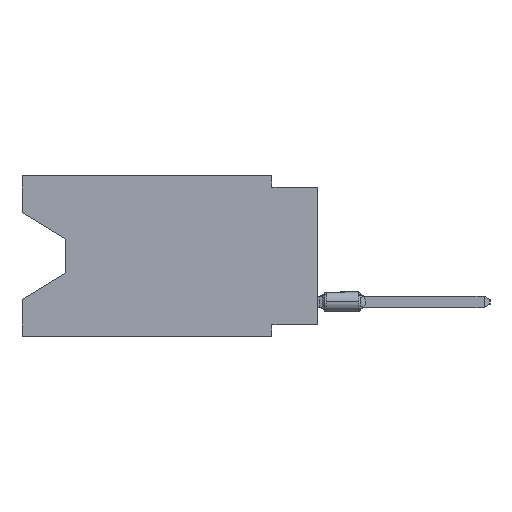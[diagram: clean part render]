
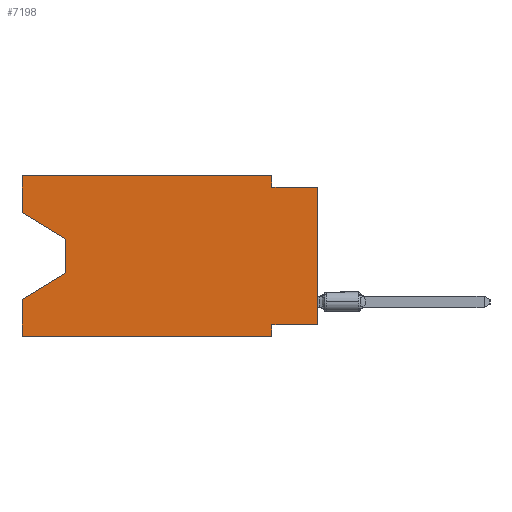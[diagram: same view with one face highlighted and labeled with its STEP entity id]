
A CAD part, left-side view. The second image highlights one B-rep face of the part: STEP entity #7198.
In plain terms, the highlighted planar face has unit normal (-1, 0, 0).
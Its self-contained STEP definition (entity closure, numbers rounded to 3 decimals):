
#345 = EDGE_LOOP ( 'NONE', ( #53610, #30509, #51926, #1708, #21597, #31156, #34441, #54796, #28527, #40102, #48692, #1842 ) ) ;
#1117 = EDGE_CURVE ( 'NONE', #38565, #13329, #57791, .T. ) ;
#1708 = ORIENTED_EDGE ( 'NONE', *, *, #26189, .F. ) ;
#1778 = CARTESIAN_POINT ( 'NONE',  ( 0., 16.383, -2.038 ) ) ;
#1842 = ORIENTED_EDGE ( 'NONE', *, *, #42715, .F. ) ;
#1951 = VECTOR ( 'NONE', #3642, 1000. ) ;
#2028 = VERTEX_POINT ( 'NONE', #43649 ) ;
#2333 = AXIS2_PLACEMENT_3D ( 'NONE', #37307, #8423, #46614 ) ;
#3642 = DIRECTION ( 'NONE',  ( 0., 0., 1. ) ) ;
#4116 = DIRECTION ( 'NONE',  ( 0., 0., -1. ) ) ;
#4872 = VERTEX_POINT ( 'NONE', #29906 ) ;
#6495 = VECTOR ( 'NONE', #46055, 1000. ) ;
#7198 = ADVANCED_FACE ( 'NONE', ( #28300 ), #37927, .F. ) ;
#8423 = DIRECTION ( 'NONE',  ( 1., 0., 0. ) ) ;
#8912 = CARTESIAN_POINT ( 'NONE',  ( 0., 0., 0. ) ) ;
#9446 = CARTESIAN_POINT ( 'NONE',  ( 0., 16.383, 0. ) ) ;
#9787 = LINE ( 'NONE', #43907, #44209 ) ;
#9845 = LINE ( 'NONE', #8912, #59745 ) ;
#10588 = DIRECTION ( 'NONE',  ( 0., 1., 0. ) ) ;
#11114 = LINE ( 'NONE', #48990, #19655 ) ;
#11750 = CARTESIAN_POINT ( 'NONE',  ( 0., 16.383, -8.89 ) ) ;
#11786 = VERTEX_POINT ( 'NONE', #42206 ) ;
#11971 = EDGE_CURVE ( 'NONE', #20358, #31687, #11114, .T. ) ;
#12134 = EDGE_CURVE ( 'NONE', #16722, #45825, #56966, .T. ) ;
#13201 = VECTOR ( 'NONE', #16327, 1000. ) ;
#13329 = VERTEX_POINT ( 'NONE', #52747 ) ;
#13511 = VERTEX_POINT ( 'NONE', #1778 ) ;
#15237 = CARTESIAN_POINT ( 'NONE',  ( 0., 0., -8.255 ) ) ;
#15670 = VECTOR ( 'NONE', #50223, 1000. ) ;
#16327 = DIRECTION ( 'NONE',  ( 0., 0.855, -0.519 ) ) ;
#16722 = VERTEX_POINT ( 'NONE', #48293 ) ;
#17622 = LINE ( 'NONE', #31303, #1951 ) ;
#18232 = DIRECTION ( 'NONE',  ( 0., 0., 1. ) ) ;
#19655 = VECTOR ( 'NONE', #35328, 1000. ) ;
#19857 = VECTOR ( 'NONE', #4116, 1000. ) ;
#20358 = VERTEX_POINT ( 'NONE', #53129 ) ;
#20748 = DIRECTION ( 'NONE',  ( 0., -1., 0. ) ) ;
#21352 = VECTOR ( 'NONE', #48007, 1000. ) ;
#21597 = ORIENTED_EDGE ( 'NONE', *, *, #58146, .T. ) ;
#22085 = VERTEX_POINT ( 'NONE', #50727 ) ;
#26189 = EDGE_CURVE ( 'NONE', #2028, #11786, #27744, .T. ) ;
#26936 = EDGE_CURVE ( 'NONE', #13511, #20358, #9787, .T. ) ;
#27744 = LINE ( 'NONE', #46372, #6495 ) ;
#27835 = CARTESIAN_POINT ( 'NONE',  ( 0., 2.54, -8.89 ) ) ;
#28300 = FACE_OUTER_BOUND ( 'NONE', #345, .T. ) ;
#28350 = CARTESIAN_POINT ( 'NONE',  ( 0., 2.54, 0. ) ) ;
#28477 = CARTESIAN_POINT ( 'NONE',  ( 0., 0., -0.635 ) ) ;
#28527 = ORIENTED_EDGE ( 'NONE', *, *, #34054, .F. ) ;
#29341 = DIRECTION ( 'NONE',  ( 0., -0.855, -0.519 ) ) ;
#29906 = CARTESIAN_POINT ( 'NONE',  ( 0., 2.54, -0.635 ) ) ;
#30509 = ORIENTED_EDGE ( 'NONE', *, *, #11971, .T. ) ;
#31156 = ORIENTED_EDGE ( 'NONE', *, *, #37331, .F. ) ;
#31157 = VECTOR ( 'NONE', #20748, 1000. ) ;
#31303 = CARTESIAN_POINT ( 'NONE',  ( 0., 16.383, 0. ) ) ;
#31687 = VERTEX_POINT ( 'NONE', #51716 ) ;
#34054 = EDGE_CURVE ( 'NONE', #4872, #22085, #38416, .T. ) ;
#34441 = ORIENTED_EDGE ( 'NONE', *, *, #1117, .F. ) ;
#35266 = CARTESIAN_POINT ( 'NONE',  ( 0., 13.97, -5.385 ) ) ;
#35328 = DIRECTION ( 'NONE',  ( 0., 0., -1. ) ) ;
#36946 = VERTEX_POINT ( 'NONE', #50960 ) ;
#37307 = CARTESIAN_POINT ( 'NONE',  ( 0., 16.383, 0. ) ) ;
#37331 = EDGE_CURVE ( 'NONE', #13329, #36946, #51745, .T. ) ;
#37927 = PLANE ( 'NONE',  #2333 ) ;
#38416 = LINE ( 'NONE', #28477, #21352 ) ;
#38565 = VERTEX_POINT ( 'NONE', #45439 ) ;
#40102 = ORIENTED_EDGE ( 'NONE', *, *, #45677, .F. ) ;
#42206 = CARTESIAN_POINT ( 'NONE',  ( 0., 16.383, -6.852 ) ) ;
#42715 = EDGE_CURVE ( 'NONE', #13511, #16722, #17622, .T. ) ;
#43649 = CARTESIAN_POINT ( 'NONE',  ( 0., 16.383, -8.89 ) ) ;
#43907 = CARTESIAN_POINT ( 'NONE',  ( 0., 16.383, -2.038 ) ) ;
#44209 = VECTOR ( 'NONE', #29341, 1000. ) ;
#45439 = CARTESIAN_POINT ( 'NONE',  ( 0., 0., -8.255 ) ) ;
#45677 = EDGE_CURVE ( 'NONE', #45825, #4872, #46655, .T. ) ;
#45825 = VERTEX_POINT ( 'NONE', #57840 ) ;
#46055 = DIRECTION ( 'NONE',  ( 0., 0., 1. ) ) ;
#46372 = CARTESIAN_POINT ( 'NONE',  ( 0., 16.383, 0. ) ) ;
#46614 = DIRECTION ( 'NONE',  ( 0., 0., -1. ) ) ;
#46655 = LINE ( 'NONE', #28350, #19857 ) ;
#46760 = DIRECTION ( 'NONE',  ( 0., 0., -1. ) ) ;
#48007 = DIRECTION ( 'NONE',  ( 0., -1., 0. ) ) ;
#48293 = CARTESIAN_POINT ( 'NONE',  ( 0., 16.383, 0. ) ) ;
#48692 = ORIENTED_EDGE ( 'NONE', *, *, #12134, .F. ) ;
#48990 = CARTESIAN_POINT ( 'NONE',  ( 0., 13.97, -3.505 ) ) ;
#50223 = DIRECTION ( 'NONE',  ( 0., -1., 0. ) ) ;
#50727 = CARTESIAN_POINT ( 'NONE',  ( 0., 0., -0.635 ) ) ;
#50960 = CARTESIAN_POINT ( 'NONE',  ( 0., 2.54, -8.89 ) ) ;
#51716 = CARTESIAN_POINT ( 'NONE',  ( 0., 13.97, -5.385 ) ) ;
#51745 = LINE ( 'NONE', #27835, #60155 ) ;
#51926 = ORIENTED_EDGE ( 'NONE', *, *, #56775, .T. ) ;
#52747 = CARTESIAN_POINT ( 'NONE',  ( 0., 2.54, -8.255 ) ) ;
#53129 = CARTESIAN_POINT ( 'NONE',  ( 0., 13.97, -3.505 ) ) ;
#53610 = ORIENTED_EDGE ( 'NONE', *, *, #26936, .T. ) ;
#54314 = LINE ( 'NONE', #11750, #31157 ) ;
#54796 = ORIENTED_EDGE ( 'NONE', *, *, #56512, .T. ) ;
#56512 = EDGE_CURVE ( 'NONE', #38565, #22085, #9845, .T. ) ;
#56775 = EDGE_CURVE ( 'NONE', #31687, #11786, #60949, .T. ) ;
#56966 = LINE ( 'NONE', #9446, #15670 ) ;
#57791 = LINE ( 'NONE', #15237, #59983 ) ;
#57840 = CARTESIAN_POINT ( 'NONE',  ( 0., 2.54, 0. ) ) ;
#58146 = EDGE_CURVE ( 'NONE', #2028, #36946, #54314, .T. ) ;
#59745 = VECTOR ( 'NONE', #18232, 1000. ) ;
#59983 = VECTOR ( 'NONE', #10588, 1000. ) ;
#60155 = VECTOR ( 'NONE', #46760, 1000. ) ;
#60949 = LINE ( 'NONE', #35266, #13201 ) ;
